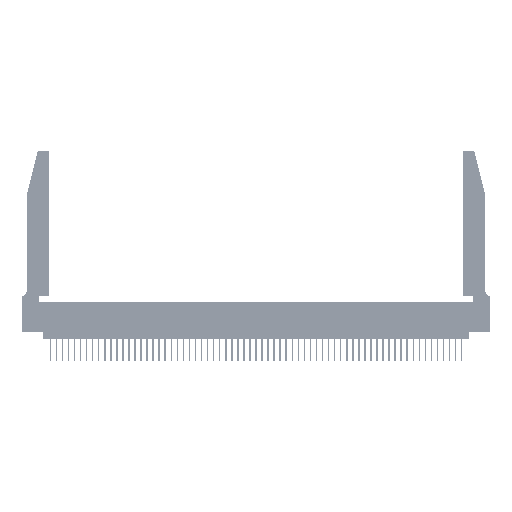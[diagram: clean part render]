
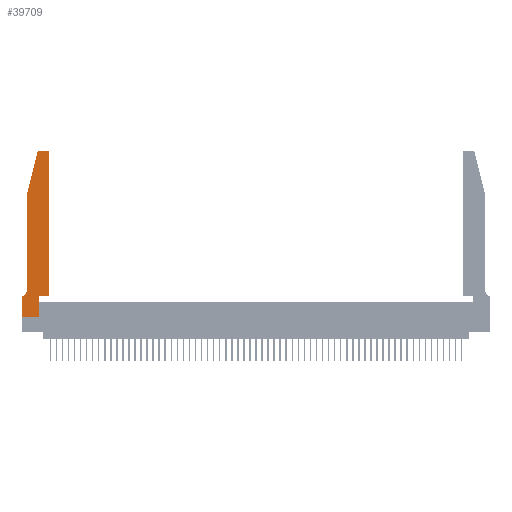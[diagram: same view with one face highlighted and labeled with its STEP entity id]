
A CAD part, top view. The second image highlights one B-rep face of the part: STEP entity #39709.
In plain terms, the highlighted planar face has unit normal (0, 0, 1).
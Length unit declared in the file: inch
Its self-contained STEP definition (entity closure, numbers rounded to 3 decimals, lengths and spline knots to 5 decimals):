
#4 = DIRECTION ( 'NONE',  ( 0., -1., 0. ) ) ;
#319 = LINE ( 'NONE', #28833, #36397 ) ;
#556 = VERTEX_POINT ( 'NONE', #27027 ) ;
#885 = CARTESIAN_POINT ( 'NONE',  ( 0., 0.35, 0.37 ) ) ;
#1935 = EDGE_CURVE ( 'NONE', #13752, #5266, #36893, .T. ) ;
#2736 = VERTEX_POINT ( 'NONE', #43103 ) ;
#4286 = VERTEX_POINT ( 'NONE', #5729 ) ;
#4895 = ORIENTED_EDGE ( 'NONE', *, *, #1935, .T. ) ;
#5266 = VERTEX_POINT ( 'NONE', #39178 ) ;
#5729 = CARTESIAN_POINT ( 'NONE',  ( 0.4505, 2.72, 0.37 ) ) ;
#6758 = VERTEX_POINT ( 'NONE', #20651 ) ;
#7152 = ORIENTED_EDGE ( 'NONE', *, *, #15829, .T. ) ;
#9117 = EDGE_CURVE ( 'NONE', #556, #36170, #319, .T. ) ;
#9990 = VECTOR ( 'NONE', #18464, 39.37008 ) ;
#11344 = LINE ( 'NONE', #52003, #9990 ) ;
#11623 = DIRECTION ( 'NONE',  ( 1., 0., 0. ) ) ;
#11916 = ORIENTED_EDGE ( 'NONE', *, *, #49729, .T. ) ;
#12985 = VECTOR ( 'NONE', #22200, 39.37008 ) ;
#13752 = VERTEX_POINT ( 'NONE', #31463 ) ;
#13841 = DIRECTION ( 'NONE',  ( -1., 0., 0. ) ) ;
#15372 = VECTOR ( 'NONE', #39171, 39.37008 ) ;
#15829 = EDGE_CURVE ( 'NONE', #25432, #31808, #48216, .T. ) ;
#16062 = VECTOR ( 'NONE', #13841, 39.37008 ) ;
#17056 = AXIS2_PLACEMENT_3D ( 'NONE', #885, #44448, #40143 ) ;
#17960 = CARTESIAN_POINT ( 'NONE',  ( 0.0755, 2., 0.37 ) ) ;
#18464 = DIRECTION ( 'NONE',  ( 0., 1., 0. ) ) ;
#18484 = EDGE_CURVE ( 'NONE', #36170, #41513, #20738, .T. ) ;
#18775 = CARTESIAN_POINT ( 'NONE',  ( 0.2605, 2.75, 0.37 ) ) ;
#19104 = CARTESIAN_POINT ( 'NONE',  ( 0.4505, 0.35, 0.37 ) ) ;
#20651 = CARTESIAN_POINT ( 'NONE',  ( 0.0055, 0.35, 0.37 ) ) ;
#20738 = LINE ( 'NONE', #50655, #15372 ) ;
#22200 = DIRECTION ( 'NONE',  ( -0.239, -0.971, 0. ) ) ;
#23033 = DIRECTION ( 'NONE',  ( -1., 0., 0. ) ) ;
#23510 = ORIENTED_EDGE ( 'NONE', *, *, #25064, .T. ) ;
#24072 = DIRECTION ( 'NONE',  ( 0., 0., -1. ) ) ;
#24078 = CARTESIAN_POINT ( 'NONE',  ( 0.2865, 0.35, 0.37 ) ) ;
#24408 = CARTESIAN_POINT ( 'NONE',  ( 0.0755, 2., 0.37 ) ) ;
#24617 = CARTESIAN_POINT ( 'NONE',  ( 0.284, 2.72, 0.37 ) ) ;
#25064 = EDGE_CURVE ( 'NONE', #2736, #556, #53286, .T. ) ;
#25432 = VERTEX_POINT ( 'NONE', #24408 ) ;
#26069 = VECTOR ( 'NONE', #37199, 39.37008 ) ;
#27027 = CARTESIAN_POINT ( 'NONE',  ( 0., 0., 0.37 ) ) ;
#27113 = ORIENTED_EDGE ( 'NONE', *, *, #33739, .T. ) ;
#28458 = ORIENTED_EDGE ( 'NONE', *, *, #48826, .T. ) ;
#28833 = CARTESIAN_POINT ( 'NONE',  ( 0., 0., 0.37 ) ) ;
#28956 = DIRECTION ( 'NONE',  ( 0., 0., 1. ) ) ;
#30297 = VERTEX_POINT ( 'NONE', #38379 ) ;
#30402 = LINE ( 'NONE', #18775, #39782 ) ;
#30592 = CARTESIAN_POINT ( 'NONE',  ( 0.4205, 2.72, 0.37 ) ) ;
#31463 = CARTESIAN_POINT ( 'NONE',  ( 0.284, 2.75, 0.37 ) ) ;
#31484 = LINE ( 'NONE', #39488, #16062 ) ;
#31808 = VERTEX_POINT ( 'NONE', #46875 ) ;
#31891 = FACE_OUTER_BOUND ( 'NONE', #55008, .T. ) ;
#32758 = VECTOR ( 'NONE', #55209, 39.37008 ) ;
#32895 = CARTESIAN_POINT ( 'NONE',  ( 0.2865, 0., 0.37 ) ) ;
#32969 = EDGE_CURVE ( 'NONE', #42382, #13752, #30402, .T. ) ;
#33005 = CIRCLE ( 'NONE', #44056, 0.07 ) ;
#33067 = ORIENTED_EDGE ( 'NONE', *, *, #35923, .T. ) ;
#33739 = EDGE_CURVE ( 'NONE', #31808, #6758, #33005, .T. ) ;
#35259 = DIRECTION ( 'NONE',  ( 1., 0., 0. ) ) ;
#35269 = CARTESIAN_POINT ( 'NONE',  ( 0.4205, 2.75, 0.37 ) ) ;
#35752 = LINE ( 'NONE', #17960, #12985 ) ;
#35923 = EDGE_CURVE ( 'NONE', #6758, #2736, #31484, .T. ) ;
#36170 = VERTEX_POINT ( 'NONE', #32895 ) ;
#36397 = VECTOR ( 'NONE', #11623, 39.37008 ) ;
#36534 = EDGE_CURVE ( 'NONE', #30297, #4286, #11344, .T. ) ;
#36893 = CIRCLE ( 'NONE', #52846, 0.03 ) ;
#37199 = DIRECTION ( 'NONE',  ( 1., 0., 0. ) ) ;
#37344 = CIRCLE ( 'NONE', #41355, 0.03 ) ;
#38148 = CARTESIAN_POINT ( 'NONE',  ( 0.0755, 2., 0.37 ) ) ;
#38379 = CARTESIAN_POINT ( 'NONE',  ( 0.4505, 0.35, 0.37 ) ) ;
#38813 = LINE ( 'NONE', #19104, #26069 ) ;
#39140 = VECTOR ( 'NONE', #4, 39.37008 ) ;
#39171 = DIRECTION ( 'NONE',  ( 0., 1., 0. ) ) ;
#39178 = CARTESIAN_POINT ( 'NONE',  ( 0.25487, 2.72718, 0.37 ) ) ;
#39488 = CARTESIAN_POINT ( 'NONE',  ( 0.0755, 0.35, 0.37 ) ) ;
#39709 = ADVANCED_FACE ( 'NONE', ( #31891 ), #52549, .T. ) ;
#39782 = VECTOR ( 'NONE', #23033, 39.37008 ) ;
#40143 = DIRECTION ( 'NONE',  ( 1., 0., 0. ) ) ;
#41355 = AXIS2_PLACEMENT_3D ( 'NONE', #30592, #51599, #35259 ) ;
#41513 = VERTEX_POINT ( 'NONE', #24078 ) ;
#42231 = DIRECTION ( 'NONE',  ( 1., 0., 0. ) ) ;
#42382 = VERTEX_POINT ( 'NONE', #35269 ) ;
#42636 = CARTESIAN_POINT ( 'NONE',  ( 0., 0., 0.37 ) ) ;
#43103 = CARTESIAN_POINT ( 'NONE',  ( 0., 0.35, 0.37 ) ) ;
#44056 = AXIS2_PLACEMENT_3D ( 'NONE', #45455, #24072, #45637 ) ;
#44420 = ORIENTED_EDGE ( 'NONE', *, *, #36534, .T. ) ;
#44448 = DIRECTION ( 'NONE',  ( 0., 0., 1. ) ) ;
#44578 = ORIENTED_EDGE ( 'NONE', *, *, #46189, .T. ) ;
#45455 = CARTESIAN_POINT ( 'NONE',  ( 0.0055, 0.42, 0.37 ) ) ;
#45637 = DIRECTION ( 'NONE',  ( -1., 0., 0. ) ) ;
#46097 = ORIENTED_EDGE ( 'NONE', *, *, #9117, .T. ) ;
#46189 = EDGE_CURVE ( 'NONE', #5266, #25432, #35752, .T. ) ;
#46875 = CARTESIAN_POINT ( 'NONE',  ( 0.0755, 0.42, 0.37 ) ) ;
#47985 = ORIENTED_EDGE ( 'NONE', *, *, #32969, .T. ) ;
#48216 = LINE ( 'NONE', #38148, #32758 ) ;
#48826 = EDGE_CURVE ( 'NONE', #41513, #30297, #38813, .T. ) ;
#49253 = ORIENTED_EDGE ( 'NONE', *, *, #18484, .T. ) ;
#49729 = EDGE_CURVE ( 'NONE', #4286, #42382, #37344, .T. ) ;
#50655 = CARTESIAN_POINT ( 'NONE',  ( 0.2865, 0.35, 0.37 ) ) ;
#51599 = DIRECTION ( 'NONE',  ( 0., 0., 1. ) ) ;
#52003 = CARTESIAN_POINT ( 'NONE',  ( 0.4505, 0.35, 0.37 ) ) ;
#52549 = PLANE ( 'NONE',  #17056 ) ;
#52846 = AXIS2_PLACEMENT_3D ( 'NONE', #24617, #28956, #42231 ) ;
#53286 = LINE ( 'NONE', #42636, #39140 ) ;
#55008 = EDGE_LOOP ( 'NONE', ( #47985, #4895, #44578, #7152, #27113, #33067, #23510, #46097, #49253, #28458, #44420, #11916 ) ) ;
#55209 = DIRECTION ( 'NONE',  ( 0., -1., 0. ) ) ;
